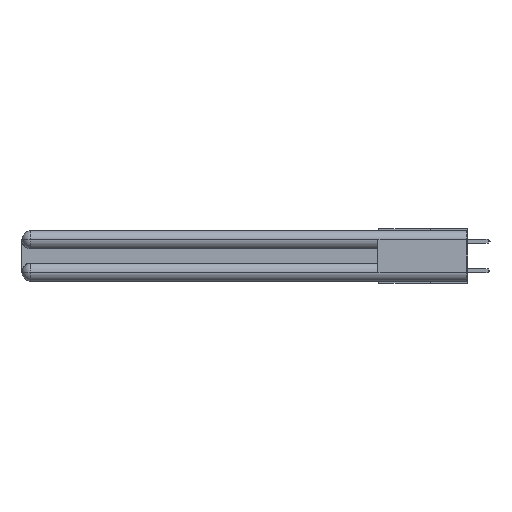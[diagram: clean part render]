
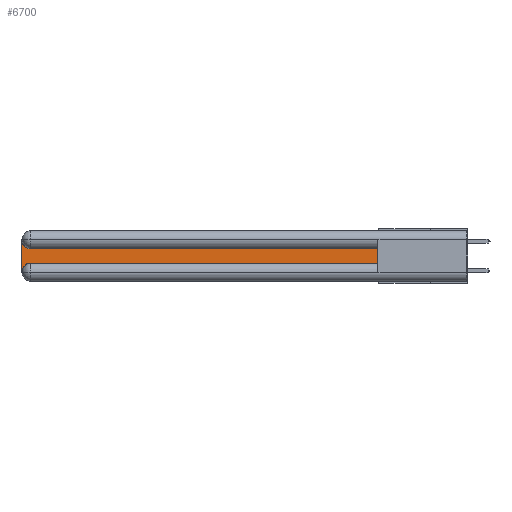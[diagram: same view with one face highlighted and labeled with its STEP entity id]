
A CAD part, left-side view. The second image highlights one B-rep face of the part: STEP entity #6700.
In plain terms, the highlighted planar face has unit normal (-1, 0, 0).
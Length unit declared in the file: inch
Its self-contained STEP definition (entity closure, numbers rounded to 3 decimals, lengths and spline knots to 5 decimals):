
#986 = EDGE_CURVE ( 'NONE', #4531, #28088, #29267, .T. ) ;
#2476 = LINE ( 'NONE', #24149, #13857 ) ;
#3111 = ORIENTED_EDGE ( 'NONE', *, *, #22928, .T. ) ;
#3250 = CARTESIAN_POINT ( 'NONE',  ( 0.075, 3., -0.2175 ) ) ;
#4078 = CARTESIAN_POINT ( 'NONE',  ( 0.075, 3., -0.0625 ) ) ;
#4531 = VERTEX_POINT ( 'NONE', #13240 ) ;
#5753 = AXIS2_PLACEMENT_3D ( 'NONE', #25729, #28280, #30709 ) ;
#6326 = DIRECTION ( 'NONE',  ( 1., 0., 0. ) ) ;
#6700 = ADVANCED_FACE ( 'NONE', ( #26245 ), #20789, .F. ) ;
#7833 = EDGE_CURVE ( 'NONE', #20636, #26166, #2476, .T. ) ;
#8185 = ORIENTED_EDGE ( 'NONE', *, *, #17486, .T. ) ;
#8353 = DIRECTION ( 'NONE',  ( 0., -1., 0. ) ) ;
#8774 = ORIENTED_EDGE ( 'NONE', *, *, #986, .T. ) ;
#9259 = EDGE_LOOP ( 'NONE', ( #13058, #21944, #8185, #18566, #8774, #3111 ) ) ;
#11199 = CARTESIAN_POINT ( 'NONE',  ( 0.075, 0.6, -0.1225 ) ) ;
#11608 = DIRECTION ( 'NONE',  ( 0., 1., 0. ) ) ;
#12959 = LINE ( 'NONE', #3250, #19701 ) ;
#13058 = ORIENTED_EDGE ( 'NONE', *, *, #7833, .T. ) ;
#13136 = CARTESIAN_POINT ( 'NONE',  ( 0.075, 3., -0.1225 ) ) ;
#13197 = DIRECTION ( 'NONE',  ( 0., 0., 1. ) ) ;
#13240 = CARTESIAN_POINT ( 'NONE',  ( 0.075, 2.94, -0.2175 ) ) ;
#13857 = VECTOR ( 'NONE', #11608, 39.37008 ) ;
#14045 = LINE ( 'NONE', #17782, #16460 ) ;
#14386 = DIRECTION ( 'NONE',  ( 0., 0., -1. ) ) ;
#14626 = CARTESIAN_POINT ( 'NONE',  ( 0.075, 3., -0.2775 ) ) ;
#15720 = DIRECTION ( 'NONE',  ( 0., 0., -1. ) ) ;
#16032 = CIRCLE ( 'NONE', #5753, 0.06 ) ;
#16460 = VECTOR ( 'NONE', #13197, 39.37008 ) ;
#17486 = EDGE_CURVE ( 'NONE', #23212, #29875, #12959, .T. ) ;
#17782 = CARTESIAN_POINT ( 'NONE',  ( 0.075, 0.6, -0.2175 ) ) ;
#18566 = ORIENTED_EDGE ( 'NONE', *, *, #18818, .T. ) ;
#18818 = EDGE_CURVE ( 'NONE', #29875, #4531, #28304, .T. ) ;
#18922 = CARTESIAN_POINT ( 'NONE',  ( 0.075, 0.6, -0.2175 ) ) ;
#19391 = VECTOR ( 'NONE', #8353, 39.37008 ) ;
#19701 = VECTOR ( 'NONE', #20550, 39.37008 ) ;
#20550 = DIRECTION ( 'NONE',  ( 0., 0., -1. ) ) ;
#20636 = VERTEX_POINT ( 'NONE', #11199 ) ;
#20789 = PLANE ( 'NONE',  #21992 ) ;
#21651 = AXIS2_PLACEMENT_3D ( 'NONE', #29567, #6326, #14386 ) ;
#21944 = ORIENTED_EDGE ( 'NONE', *, *, #31452, .T. ) ;
#21992 = AXIS2_PLACEMENT_3D ( 'NONE', #13136, #30866, #15720 ) ;
#22928 = EDGE_CURVE ( 'NONE', #28088, #20636, #14045, .T. ) ;
#23212 = VERTEX_POINT ( 'NONE', #4078 ) ;
#23705 = CARTESIAN_POINT ( 'NONE',  ( 0.075, 2.94, -0.1225 ) ) ;
#24149 = CARTESIAN_POINT ( 'NONE',  ( 0.075, 0.6, -0.1225 ) ) ;
#25729 = CARTESIAN_POINT ( 'NONE',  ( 0.075, 2.94, -0.0625 ) ) ;
#26166 = VERTEX_POINT ( 'NONE', #23705 ) ;
#26245 = FACE_OUTER_BOUND ( 'NONE', #9259, .T. ) ;
#28088 = VERTEX_POINT ( 'NONE', #18922 ) ;
#28280 = DIRECTION ( 'NONE',  ( 1., 0., 0. ) ) ;
#28304 = CIRCLE ( 'NONE', #21651, 0.06 ) ;
#28615 = CARTESIAN_POINT ( 'NONE',  ( 0.075, 0.6, -0.2175 ) ) ;
#29267 = LINE ( 'NONE', #28615, #19391 ) ;
#29567 = CARTESIAN_POINT ( 'NONE',  ( 0.075, 2.94, -0.2775 ) ) ;
#29875 = VERTEX_POINT ( 'NONE', #14626 ) ;
#30709 = DIRECTION ( 'NONE',  ( 0., 0., -1. ) ) ;
#30866 = DIRECTION ( 'NONE',  ( 1., 0., 0. ) ) ;
#31452 = EDGE_CURVE ( 'NONE', #26166, #23212, #16032, .T. ) ;
